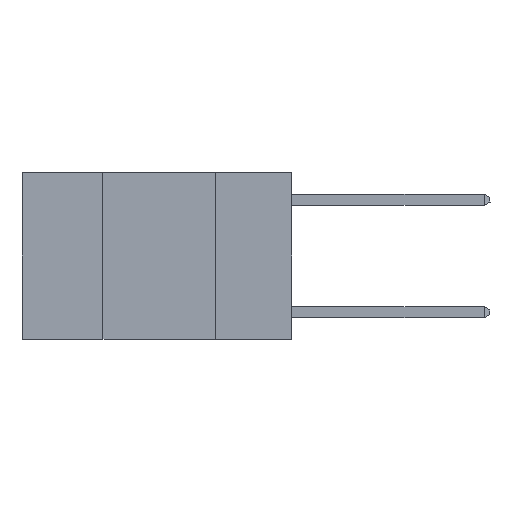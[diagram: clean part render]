
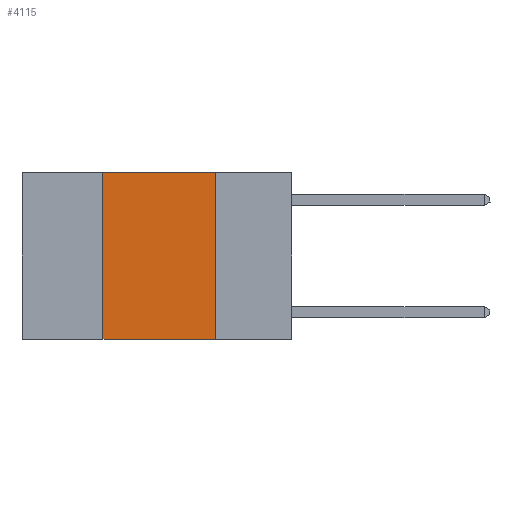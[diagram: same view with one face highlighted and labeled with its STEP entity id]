
A CAD part, left-side view. The second image highlights one B-rep face of the part: STEP entity #4115.
In plain terms, the highlighted planar face has unit normal (-1, 0, 0).
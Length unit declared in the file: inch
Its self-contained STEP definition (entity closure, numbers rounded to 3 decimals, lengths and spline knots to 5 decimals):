
#884 = LINE ( 'NONE', #4463, #17267 ) ;
#1695 = DIRECTION ( 'NONE',  ( 0., 0., -1. ) ) ;
#2717 = ORIENTED_EDGE ( 'NONE', *, *, #17114, .F. ) ;
#4115 = ADVANCED_FACE ( 'NONE', ( #20779 ), #26266, .F. ) ;
#4463 = CARTESIAN_POINT ( 'NONE',  ( 0., 0.17, 0. ) ) ;
#4509 = VECTOR ( 'NONE', #5399, 39.37008 ) ;
#5399 = DIRECTION ( 'NONE',  ( 0., -1., 0. ) ) ;
#6939 = VERTEX_POINT ( 'NONE', #19377 ) ;
#7090 = EDGE_CURVE ( 'NONE', #15498, #18506, #20963, .T. ) ;
#8187 = ORIENTED_EDGE ( 'NONE', *, *, #14879, .F. ) ;
#10455 = AXIS2_PLACEMENT_3D ( 'NONE', #18044, #13983, #1695 ) ;
#12108 = EDGE_LOOP ( 'NONE', ( #18512, #2717, #8187, #19786 ) ) ;
#12602 = VERTEX_POINT ( 'NONE', #24949 ) ;
#13487 = LINE ( 'NONE', #21782, #18969 ) ;
#13983 = DIRECTION ( 'NONE',  ( 1., 0., 0. ) ) ;
#14879 = EDGE_CURVE ( 'NONE', #15498, #12602, #18453, .T. ) ;
#15498 = VERTEX_POINT ( 'NONE', #26209 ) ;
#15846 = CARTESIAN_POINT ( 'NONE',  ( 0., 0.42, 0. ) ) ;
#17114 = EDGE_CURVE ( 'NONE', #12602, #6939, #13487, .T. ) ;
#17267 = VECTOR ( 'NONE', #24998, 39.37008 ) ;
#18044 = CARTESIAN_POINT ( 'NONE',  ( 0., 0.6, 0. ) ) ;
#18453 = LINE ( 'NONE', #15846, #22618 ) ;
#18506 = VERTEX_POINT ( 'NONE', #24129 ) ;
#18512 = ORIENTED_EDGE ( 'NONE', *, *, #19543, .F. ) ;
#18969 = VECTOR ( 'NONE', #23839, 39.37008 ) ;
#19377 = CARTESIAN_POINT ( 'NONE',  ( 0., 0.17, 0. ) ) ;
#19543 = EDGE_CURVE ( 'NONE', #6939, #18506, #884, .T. ) ;
#19786 = ORIENTED_EDGE ( 'NONE', *, *, #7090, .T. ) ;
#19964 = DIRECTION ( 'NONE',  ( 0., 0., 1. ) ) ;
#20779 = FACE_OUTER_BOUND ( 'NONE', #12108, .T. ) ;
#20963 = LINE ( 'NONE', #25986, #4509 ) ;
#21782 = CARTESIAN_POINT ( 'NONE',  ( 0., 0.6, 0. ) ) ;
#22618 = VECTOR ( 'NONE', #19964, 39.37008 ) ;
#23839 = DIRECTION ( 'NONE',  ( 0., -1., 0. ) ) ;
#24129 = CARTESIAN_POINT ( 'NONE',  ( 0., 0.17, -0.37 ) ) ;
#24949 = CARTESIAN_POINT ( 'NONE',  ( 0., 0.42, 0. ) ) ;
#24998 = DIRECTION ( 'NONE',  ( 0., 0., -1. ) ) ;
#25986 = CARTESIAN_POINT ( 'NONE',  ( 0., 0.6, -0.37 ) ) ;
#26209 = CARTESIAN_POINT ( 'NONE',  ( 0., 0.42, -0.37 ) ) ;
#26266 = PLANE ( 'NONE',  #10455 ) ;
